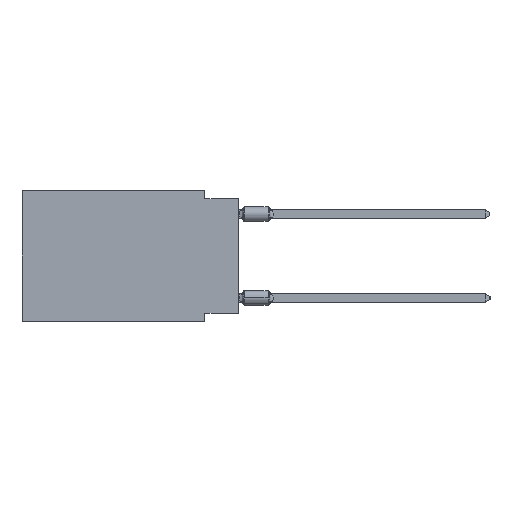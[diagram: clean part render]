
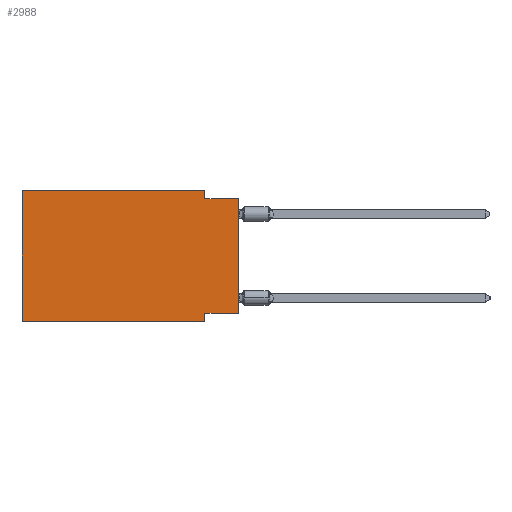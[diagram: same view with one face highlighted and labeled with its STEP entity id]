
A CAD part, left-side view. The second image highlights one B-rep face of the part: STEP entity #2988.
In plain terms, the highlighted planar face has unit normal (-1, 0, 0).
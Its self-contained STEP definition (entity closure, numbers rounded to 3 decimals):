
#10 = VECTOR ( 'NONE', #3677, 1000. ) ;
#179 = DIRECTION ( 'NONE',  ( 0., -1., 0. ) ) ;
#858 = ORIENTED_EDGE ( 'NONE', *, *, #8624, .T. ) ;
#1098 = DIRECTION ( 'NONE',  ( 0., 0., 1. ) ) ;
#1127 = ORIENTED_EDGE ( 'NONE', *, *, #8683, .F. ) ;
#2216 = CARTESIAN_POINT ( 'NONE',  ( 0., 16.383, -9.906 ) ) ;
#2222 = PLANE ( 'NONE',  #18820 ) ;
#2761 = VERTEX_POINT ( 'NONE', #26387 ) ;
#2988 = ADVANCED_FACE ( 'NONE', ( #39742 ), #2222, .F. ) ;
#3309 = CARTESIAN_POINT ( 'NONE',  ( 0., 0., -0.635 ) ) ;
#3677 = DIRECTION ( 'NONE',  ( 0., 0., 1. ) ) ;
#4730 = VECTOR ( 'NONE', #14427, 1000. ) ;
#5117 = ORIENTED_EDGE ( 'NONE', *, *, #17045, .F. ) ;
#5875 = DIRECTION ( 'NONE',  ( 0., 0., -1. ) ) ;
#6825 = CARTESIAN_POINT ( 'NONE',  ( 0., 2.54, -9.906 ) ) ;
#7257 = VERTEX_POINT ( 'NONE', #31737 ) ;
#7728 = CARTESIAN_POINT ( 'NONE',  ( 0., 2.54, 0. ) ) ;
#8624 = EDGE_CURVE ( 'NONE', #7257, #28692, #32421, .T. ) ;
#8683 = EDGE_CURVE ( 'NONE', #2761, #41798, #25114, .T. ) ;
#8765 = ORIENTED_EDGE ( 'NONE', *, *, #32542, .F. ) ;
#9143 = EDGE_CURVE ( 'NONE', #33133, #21375, #9684, .T. ) ;
#9384 = CARTESIAN_POINT ( 'NONE',  ( 0., 2.54, -0.635 ) ) ;
#9684 = LINE ( 'NONE', #33031, #10912 ) ;
#10757 = CARTESIAN_POINT ( 'NONE',  ( 0., 16.383, 0. ) ) ;
#10912 = VECTOR ( 'NONE', #44444, 1000. ) ;
#11700 = VERTEX_POINT ( 'NONE', #44876 ) ;
#14427 = DIRECTION ( 'NONE',  ( 0., -1., 0. ) ) ;
#14844 = CARTESIAN_POINT ( 'NONE',  ( 0., 2.54, -9.271 ) ) ;
#17045 = EDGE_CURVE ( 'NONE', #7257, #23010, #36329, .T. ) ;
#17320 = DIRECTION ( 'NONE',  ( 0., 1., 0. ) ) ;
#17988 = EDGE_CURVE ( 'NONE', #33133, #11700, #45048, .T. ) ;
#18345 = EDGE_CURVE ( 'NONE', #41798, #28692, #20295, .T. ) ;
#18820 = AXIS2_PLACEMENT_3D ( 'NONE', #36531, #43621, #5875 ) ;
#20295 = LINE ( 'NONE', #34235, #37982 ) ;
#21375 = VERTEX_POINT ( 'NONE', #36462 ) ;
#21684 = DIRECTION ( 'NONE',  ( 0., 0., -1. ) ) ;
#21820 = ORIENTED_EDGE ( 'NONE', *, *, #22421, .F. ) ;
#21940 = EDGE_LOOP ( 'NONE', ( #858, #24957, #1127, #8765, #44527, #36045, #21820, #5117 ) ) ;
#21967 = LINE ( 'NONE', #25392, #4730 ) ;
#22421 = EDGE_CURVE ( 'NONE', #23010, #21375, #38141, .T. ) ;
#23010 = VERTEX_POINT ( 'NONE', #14844 ) ;
#24957 = ORIENTED_EDGE ( 'NONE', *, *, #18345, .F. ) ;
#25114 = LINE ( 'NONE', #7728, #29161 ) ;
#25392 = CARTESIAN_POINT ( 'NONE',  ( 0., 16.383, 0. ) ) ;
#26387 = CARTESIAN_POINT ( 'NONE',  ( 0., 2.54, 0. ) ) ;
#27368 = CARTESIAN_POINT ( 'NONE',  ( 0., 0., -9.271 ) ) ;
#28692 = VERTEX_POINT ( 'NONE', #3309 ) ;
#29161 = VECTOR ( 'NONE', #21684, 1000. ) ;
#29177 = VECTOR ( 'NONE', #41346, 1000. ) ;
#31737 = CARTESIAN_POINT ( 'NONE',  ( 0., 0., -9.271 ) ) ;
#32097 = VECTOR ( 'NONE', #17320, 1000. ) ;
#32421 = LINE ( 'NONE', #43164, #40827 ) ;
#32542 = EDGE_CURVE ( 'NONE', #11700, #2761, #21967, .T. ) ;
#33031 = CARTESIAN_POINT ( 'NONE',  ( 0., 16.383, -9.906 ) ) ;
#33133 = VERTEX_POINT ( 'NONE', #2216 ) ;
#34235 = CARTESIAN_POINT ( 'NONE',  ( 0., 0., -0.635 ) ) ;
#36045 = ORIENTED_EDGE ( 'NONE', *, *, #9143, .T. ) ;
#36329 = LINE ( 'NONE', #27368, #32097 ) ;
#36462 = CARTESIAN_POINT ( 'NONE',  ( 0., 2.54, -9.906 ) ) ;
#36531 = CARTESIAN_POINT ( 'NONE',  ( 0., 16.383, 0. ) ) ;
#37982 = VECTOR ( 'NONE', #179, 1000. ) ;
#38141 = LINE ( 'NONE', #6825, #29177 ) ;
#39742 = FACE_OUTER_BOUND ( 'NONE', #21940, .T. ) ;
#40827 = VECTOR ( 'NONE', #1098, 1000. ) ;
#41346 = DIRECTION ( 'NONE',  ( 0., 0., -1. ) ) ;
#41798 = VERTEX_POINT ( 'NONE', #9384 ) ;
#43164 = CARTESIAN_POINT ( 'NONE',  ( 0., 0., 0. ) ) ;
#43621 = DIRECTION ( 'NONE',  ( 1., 0., 0. ) ) ;
#44444 = DIRECTION ( 'NONE',  ( 0., -1., 0. ) ) ;
#44527 = ORIENTED_EDGE ( 'NONE', *, *, #17988, .F. ) ;
#44876 = CARTESIAN_POINT ( 'NONE',  ( 0., 16.383, 0. ) ) ;
#45048 = LINE ( 'NONE', #10757, #10 ) ;
